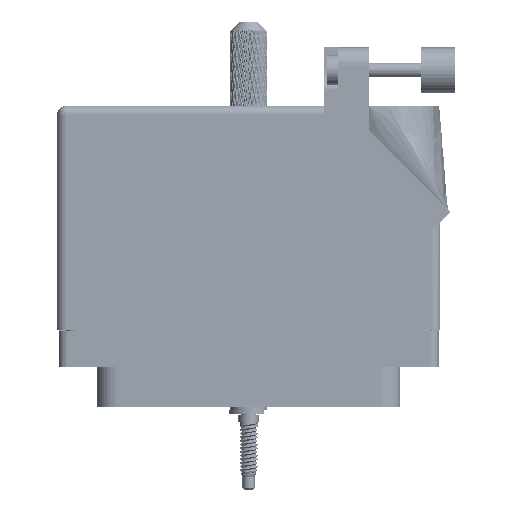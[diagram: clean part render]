
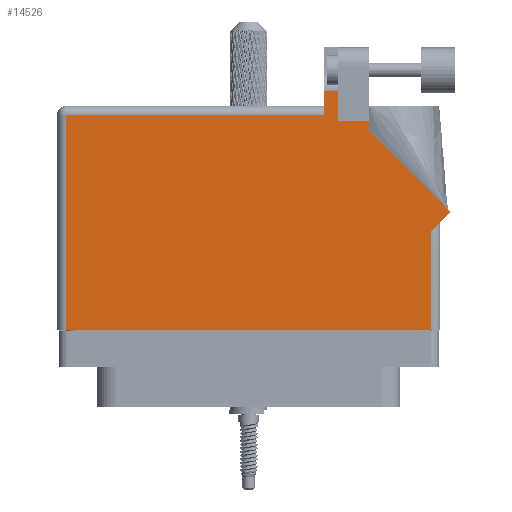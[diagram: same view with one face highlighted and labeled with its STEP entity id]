
A CAD part, front view. The second image highlights one B-rep face of the part: STEP entity #14526.
In plain terms, the highlighted face is planar.
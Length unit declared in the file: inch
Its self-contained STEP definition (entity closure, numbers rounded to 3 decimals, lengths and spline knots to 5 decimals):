
#59 = CARTESIAN_POINT ( 'NONE',  ( 0.82, 1.33, 0.455 ) ) ;
#1323 = ORIENTED_EDGE ( 'NONE', *, *, #55746, .T. ) ;
#2337 = ORIENTED_EDGE ( 'NONE', *, *, #53615, .T. ) ;
#4605 = DIRECTION ( 'NONE',  ( 0.707, 0.707, 0. ) ) ;
#5402 = DIRECTION ( 'NONE',  ( 0., 0., -1. ) ) ;
#6234 = VECTOR ( 'NONE', #100508, 39.37008 ) ;
#11551 = CARTESIAN_POINT ( 'NONE',  ( -1.244, -0.1, 0.455 ) ) ;
#14526 = ADVANCED_FACE ( 'NONE', ( #69777 ), #31715, .F. ) ;
#15394 = CARTESIAN_POINT ( 'NONE',  ( 0.82, 1.26442, 0.455 ) ) ;
#15463 = EDGE_CURVE ( 'NONE', #25040, #98209, #99499, .T. ) ;
#17496 = VECTOR ( 'NONE', #103138, 39.37008 ) ;
#21140 = DIRECTION ( 'NONE',  ( 0., -1., 0. ) ) ;
#24121 = CARTESIAN_POINT ( 'NONE',  ( 1.244, 0.637, 0.455 ) ) ;
#24803 = VECTOR ( 'NONE', #81220, 39.37008 ) ;
#25040 = VERTEX_POINT ( 'NONE', #62483 ) ;
#25622 = EDGE_LOOP ( 'NONE', ( #90457, #34253, #106248, #113283, #2337, #51064, #62535, #116176, #49849, #1323, #68378 ) ) ;
#26195 = CARTESIAN_POINT ( 'NONE',  ( 0.513, 1.43, 0.455 ) ) ;
#30501 = LINE ( 'NONE', #64391, #6234 ) ;
#31715 = PLANE ( 'NONE',  #102855 ) ;
#32664 = CARTESIAN_POINT ( 'NONE',  ( 1.244, -0.1, 0.455 ) ) ;
#33119 = LINE ( 'NONE', #11551, #74490 ) ;
#34253 = ORIENTED_EDGE ( 'NONE', *, *, #15463, .T. ) ;
#36354 = LINE ( 'NONE', #26195, #24803 ) ;
#41985 = LINE ( 'NONE', #60021, #46246 ) ;
#46246 = VECTOR ( 'NONE', #4605, 39.37008 ) ;
#49005 = CARTESIAN_POINT ( 'NONE',  ( 1.37671, 0.70771, 0.455 ) ) ;
#49849 = ORIENTED_EDGE ( 'NONE', *, *, #101350, .T. ) ;
#50893 = DIRECTION ( 'NONE',  ( -1., 0., 0. ) ) ;
#51064 = ORIENTED_EDGE ( 'NONE', *, *, #106355, .T. ) ;
#51148 = EDGE_CURVE ( 'NONE', #92581, #65442, #30501, .T. ) ;
#53615 = EDGE_CURVE ( 'NONE', #65442, #109496, #33119, .T. ) ;
#54868 = CARTESIAN_POINT ( 'NONE',  ( 0.607, 1.33, 0.455 ) ) ;
#55368 = VECTOR ( 'NONE', #112719, 39.37008 ) ;
#55746 = EDGE_CURVE ( 'NONE', #61975, #90108, #116987, .T. ) ;
#59606 = CARTESIAN_POINT ( 'NONE',  ( -1.244, 1.368, 0.455 ) ) ;
#60021 = CARTESIAN_POINT ( 'NONE',  ( 1.306, 0.637, 0.455 ) ) ;
#61975 = VERTEX_POINT ( 'NONE', #15394 ) ;
#62483 = CARTESIAN_POINT ( 'NONE',  ( 0.607, 1.5315, 0.455 ) ) ;
#62535 = ORIENTED_EDGE ( 'NONE', *, *, #108819, .T. ) ;
#63788 = LINE ( 'NONE', #24121, #72365 ) ;
#64098 = EDGE_CURVE ( 'NONE', #76030, #25040, #100450, .T. ) ;
#64391 = CARTESIAN_POINT ( 'NONE',  ( -1.306, 1.368, 0.455 ) ) ;
#65017 = CARTESIAN_POINT ( 'NONE',  ( -1.306, -0.1, 0.455 ) ) ;
#65442 = VERTEX_POINT ( 'NONE', #59606 ) ;
#65735 = VECTOR ( 'NONE', #93589, 39.37008 ) ;
#67455 = CARTESIAN_POINT ( 'NONE',  ( 0.82, 1.26442, 0.455 ) ) ;
#68378 = ORIENTED_EDGE ( 'NONE', *, *, #91575, .T. ) ;
#69514 = EDGE_CURVE ( 'NONE', #95719, #81345, #41985, .T. ) ;
#69777 = FACE_OUTER_BOUND ( 'NONE', #25622, .T. ) ;
#72095 = CARTESIAN_POINT ( 'NONE',  ( 1.244, 0.575, 0.455 ) ) ;
#72110 = CARTESIAN_POINT ( 'NONE',  ( 0.82, 1.33, 0.455 ) ) ;
#72365 = VECTOR ( 'NONE', #87481, 39.37008 ) ;
#74039 = LINE ( 'NONE', #65017, #95323 ) ;
#74126 = DIRECTION ( 'NONE',  ( 1., 0., 0. ) ) ;
#74490 = VECTOR ( 'NONE', #21140, 39.37008 ) ;
#76030 = VERTEX_POINT ( 'NONE', #54868 ) ;
#76311 = VECTOR ( 'NONE', #110374, 39.37008 ) ;
#77992 = CARTESIAN_POINT ( 'NONE',  ( 1.37671, 0.70771, 0.455 ) ) ;
#80548 = CARTESIAN_POINT ( 'NONE',  ( -1.244, -0.1, 0.455 ) ) ;
#81220 = DIRECTION ( 'NONE',  ( 0., -1., 0. ) ) ;
#81345 = VERTEX_POINT ( 'NONE', #77992 ) ;
#84268 = LINE ( 'NONE', #59, #92784 ) ;
#84851 = CARTESIAN_POINT ( 'NONE',  ( 0.93777, 1.5315, 0.455 ) ) ;
#87481 = DIRECTION ( 'NONE',  ( 0., 1., 0. ) ) ;
#90108 = VERTEX_POINT ( 'NONE', #72110 ) ;
#90457 = ORIENTED_EDGE ( 'NONE', *, *, #64098, .T. ) ;
#91575 = EDGE_CURVE ( 'NONE', #90108, #76030, #84268, .T. ) ;
#92581 = VERTEX_POINT ( 'NONE', #116088 ) ;
#92784 = VECTOR ( 'NONE', #108090, 39.37008 ) ;
#93589 = DIRECTION ( 'NONE',  ( 0., 1., 0. ) ) ;
#95323 = VECTOR ( 'NONE', #74126, 39.37008 ) ;
#95719 = VERTEX_POINT ( 'NONE', #72095 ) ;
#98209 = VERTEX_POINT ( 'NONE', #104287 ) ;
#99499 = LINE ( 'NONE', #84851, #55368 ) ;
#100450 = LINE ( 'NONE', #100776, #76311 ) ;
#100508 = DIRECTION ( 'NONE',  ( -1., 0., 0. ) ) ;
#100776 = CARTESIAN_POINT ( 'NONE',  ( 0.607, 1.33, 0.455 ) ) ;
#101350 = EDGE_CURVE ( 'NONE', #81345, #61975, #117377, .T. ) ;
#102855 = AXIS2_PLACEMENT_3D ( 'NONE', #105452, #5402, #50893 ) ;
#103138 = DIRECTION ( 'NONE',  ( -0.707, 0.707, 0. ) ) ;
#104287 = CARTESIAN_POINT ( 'NONE',  ( 0.513, 1.5315, 0.455 ) ) ;
#105452 = CARTESIAN_POINT ( 'NONE',  ( -1.306, 1.43, 0.455 ) ) ;
#106248 = ORIENTED_EDGE ( 'NONE', *, *, #111832, .T. ) ;
#106265 = VERTEX_POINT ( 'NONE', #32664 ) ;
#106355 = EDGE_CURVE ( 'NONE', #109496, #106265, #74039, .T. ) ;
#108090 = DIRECTION ( 'NONE',  ( -1., 0., 0. ) ) ;
#108819 = EDGE_CURVE ( 'NONE', #106265, #95719, #63788, .T. ) ;
#109496 = VERTEX_POINT ( 'NONE', #80548 ) ;
#110374 = DIRECTION ( 'NONE',  ( 0., 1., 0. ) ) ;
#111832 = EDGE_CURVE ( 'NONE', #98209, #92581, #36354, .T. ) ;
#112719 = DIRECTION ( 'NONE',  ( -1., 0., 0. ) ) ;
#113283 = ORIENTED_EDGE ( 'NONE', *, *, #51148, .T. ) ;
#116088 = CARTESIAN_POINT ( 'NONE',  ( 0.513, 1.368, 0.455 ) ) ;
#116176 = ORIENTED_EDGE ( 'NONE', *, *, #69514, .T. ) ;
#116987 = LINE ( 'NONE', #67455, #65735 ) ;
#117377 = LINE ( 'NONE', #49005, #17496 ) ;
